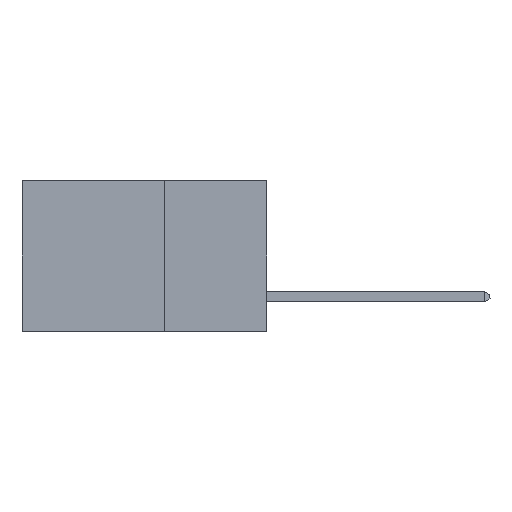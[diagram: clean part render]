
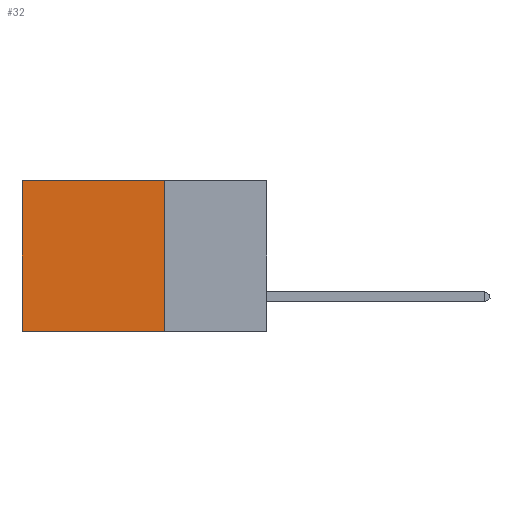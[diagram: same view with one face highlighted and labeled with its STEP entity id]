
A CAD part, left-side view. The second image highlights one B-rep face of the part: STEP entity #32.
In plain terms, the highlighted planar face has unit normal (-1, 0, 0).
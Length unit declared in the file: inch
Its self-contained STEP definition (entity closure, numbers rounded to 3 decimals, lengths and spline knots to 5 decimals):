
#32 = ADVANCED_FACE ( 'NONE', ( #13232 ), #6648, .F. ) ;
#902 = ORIENTED_EDGE ( 'NONE', *, *, #24323, .F. ) ;
#2210 = VECTOR ( 'NONE', #17042, 39.37008 ) ;
#4160 = DIRECTION ( 'NONE',  ( 0., 0., -1. ) ) ;
#4954 = EDGE_CURVE ( 'NONE', #7508, #24019, #5539, .T. ) ;
#5539 = LINE ( 'NONE', #23016, #20523 ) ;
#6648 = PLANE ( 'NONE',  #18928 ) ;
#7124 = CARTESIAN_POINT ( 'NONE',  ( 0.2875, 0.6, -0.37 ) ) ;
#7352 = CARTESIAN_POINT ( 'NONE',  ( 0.2875, 0.25, 0. ) ) ;
#7508 = VERTEX_POINT ( 'NONE', #24973 ) ;
#8135 = LINE ( 'NONE', #7352, #2210 ) ;
#8399 = VERTEX_POINT ( 'NONE', #22206 ) ;
#9992 = LINE ( 'NONE', #11993, #14520 ) ;
#11993 = CARTESIAN_POINT ( 'NONE',  ( 0.2875, 0.25, 0. ) ) ;
#12377 = CARTESIAN_POINT ( 'NONE',  ( 0.2875, 0.25, -0.37 ) ) ;
#13232 = FACE_OUTER_BOUND ( 'NONE', #20089, .T. ) ;
#14520 = VECTOR ( 'NONE', #4160, 39.37008 ) ;
#15610 = CARTESIAN_POINT ( 'NONE',  ( 0.2875, 0.25, -0.37 ) ) ;
#16243 = DIRECTION ( 'NONE',  ( 0., 0., -1. ) ) ;
#16282 = ORIENTED_EDGE ( 'NONE', *, *, #4954, .T. ) ;
#17042 = DIRECTION ( 'NONE',  ( 0., 1., 0. ) ) ;
#17804 = DIRECTION ( 'NONE',  ( 1., 0., 0. ) ) ;
#18416 = VERTEX_POINT ( 'NONE', #12377 ) ;
#18928 = AXIS2_PLACEMENT_3D ( 'NONE', #19100, #17804, #16243 ) ;
#19100 = CARTESIAN_POINT ( 'NONE',  ( 0.2875, 0.25, 0. ) ) ;
#19595 = VECTOR ( 'NONE', #21440, 39.37008 ) ;
#20089 = EDGE_LOOP ( 'NONE', ( #16282, #23378, #902, #25284 ) ) ;
#20523 = VECTOR ( 'NONE', #24920, 39.37008 ) ;
#21161 = EDGE_CURVE ( 'NONE', #18416, #24019, #23604, .T. ) ;
#21440 = DIRECTION ( 'NONE',  ( 0., 1., 0. ) ) ;
#22206 = CARTESIAN_POINT ( 'NONE',  ( 0.2875, 0.25, 0. ) ) ;
#23016 = CARTESIAN_POINT ( 'NONE',  ( 0.2875, 0.6, 0. ) ) ;
#23378 = ORIENTED_EDGE ( 'NONE', *, *, #21161, .F. ) ;
#23604 = LINE ( 'NONE', #15610, #19595 ) ;
#24019 = VERTEX_POINT ( 'NONE', #7124 ) ;
#24323 = EDGE_CURVE ( 'NONE', #8399, #18416, #9992, .T. ) ;
#24706 = EDGE_CURVE ( 'NONE', #8399, #7508, #8135, .T. ) ;
#24920 = DIRECTION ( 'NONE',  ( 0., 0., -1. ) ) ;
#24973 = CARTESIAN_POINT ( 'NONE',  ( 0.2875, 0.6, 0. ) ) ;
#25284 = ORIENTED_EDGE ( 'NONE', *, *, #24706, .T. ) ;
